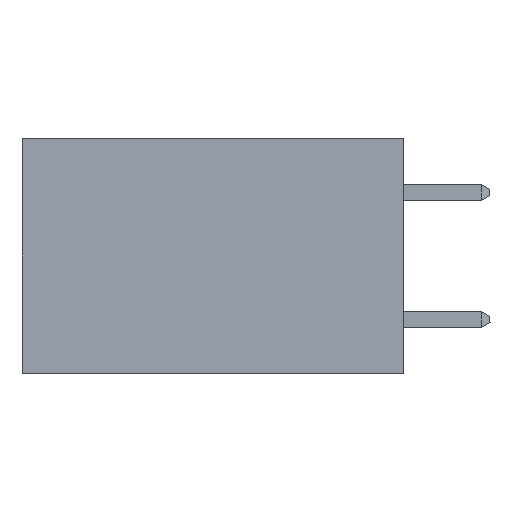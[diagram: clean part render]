
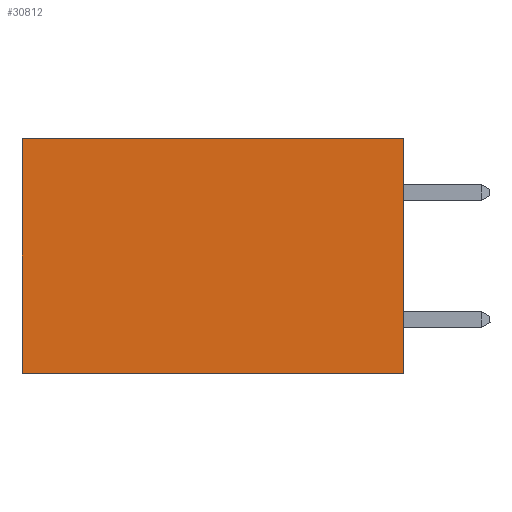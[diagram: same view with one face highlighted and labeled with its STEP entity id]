
A CAD part, left-side view. The second image highlights one B-rep face of the part: STEP entity #30812.
In plain terms, the highlighted planar face has unit normal (-1, 0, 0).
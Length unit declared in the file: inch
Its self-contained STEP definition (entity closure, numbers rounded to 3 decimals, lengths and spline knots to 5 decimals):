
#636 = LINE ( 'NONE', #20253, #21174 ) ;
#5916 = EDGE_CURVE ( 'NONE', #31765, #15595, #15715, .T. ) ;
#6151 = CARTESIAN_POINT ( 'NONE',  ( 0.2875, 0.6, -0.37 ) ) ;
#6843 = DIRECTION ( 'NONE',  ( 0., 0., -1. ) ) ;
#7361 = ORIENTED_EDGE ( 'NONE', *, *, #21997, .F. ) ;
#9056 = VERTEX_POINT ( 'NONE', #19735 ) ;
#9151 = VECTOR ( 'NONE', #18736, 39.37008 ) ;
#9284 = AXIS2_PLACEMENT_3D ( 'NONE', #20734, #9652, #29088 ) ;
#9652 = DIRECTION ( 'NONE',  ( 1., 0., 0. ) ) ;
#11529 = VECTOR ( 'NONE', #6843, 39.37008 ) ;
#12030 = ORIENTED_EDGE ( 'NONE', *, *, #15401, .F. ) ;
#12105 = ORIENTED_EDGE ( 'NONE', *, *, #5916, .T. ) ;
#12323 = PLANE ( 'NONE',  #9284 ) ;
#12334 = CARTESIAN_POINT ( 'NONE',  ( 0.2875, 0.6, 0. ) ) ;
#13178 = CARTESIAN_POINT ( 'NONE',  ( 0.2875, 0., -0.37 ) ) ;
#14105 = ORIENTED_EDGE ( 'NONE', *, *, #33561, .T. ) ;
#14395 = CARTESIAN_POINT ( 'NONE',  ( 0.2875, 0.6, 0. ) ) ;
#14667 = DIRECTION ( 'NONE',  ( 0., 0., -1. ) ) ;
#15401 = EDGE_CURVE ( 'NONE', #9056, #26576, #27694, .T. ) ;
#15595 = VERTEX_POINT ( 'NONE', #14395 ) ;
#15715 = LINE ( 'NONE', #35261, #9151 ) ;
#16167 = EDGE_LOOP ( 'NONE', ( #14105, #12030, #7361, #12105 ) ) ;
#16954 = FACE_OUTER_BOUND ( 'NONE', #16167, .T. ) ;
#18736 = DIRECTION ( 'NONE',  ( 0., 1., 0. ) ) ;
#19735 = CARTESIAN_POINT ( 'NONE',  ( 0.2875, 0., -0.37 ) ) ;
#20253 = CARTESIAN_POINT ( 'NONE',  ( 0.2875, 0., 0. ) ) ;
#20315 = VECTOR ( 'NONE', #32560, 39.37008 ) ;
#20734 = CARTESIAN_POINT ( 'NONE',  ( 0.2875, 0., 0. ) ) ;
#21174 = VECTOR ( 'NONE', #14667, 39.37008 ) ;
#21997 = EDGE_CURVE ( 'NONE', #31765, #9056, #636, .T. ) ;
#26576 = VERTEX_POINT ( 'NONE', #6151 ) ;
#27694 = LINE ( 'NONE', #13178, #20315 ) ;
#29088 = DIRECTION ( 'NONE',  ( 0., 0., -1. ) ) ;
#30812 = ADVANCED_FACE ( 'NONE', ( #16954 ), #12323, .F. ) ;
#31765 = VERTEX_POINT ( 'NONE', #32889 ) ;
#32560 = DIRECTION ( 'NONE',  ( 0., 1., 0. ) ) ;
#32889 = CARTESIAN_POINT ( 'NONE',  ( 0.2875, 0., 0. ) ) ;
#33561 = EDGE_CURVE ( 'NONE', #15595, #26576, #33627, .T. ) ;
#33627 = LINE ( 'NONE', #12334, #11529 ) ;
#35261 = CARTESIAN_POINT ( 'NONE',  ( 0.2875, 0., 0. ) ) ;
